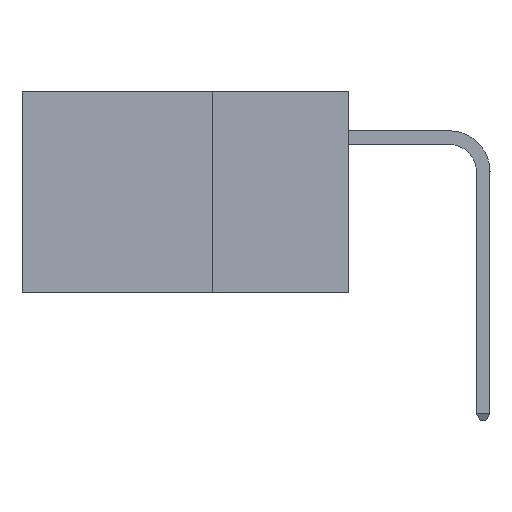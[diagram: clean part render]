
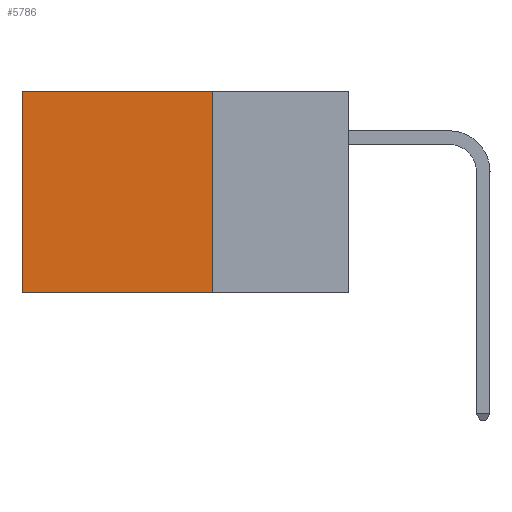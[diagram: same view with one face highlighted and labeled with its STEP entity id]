
A CAD part, left-side view. The second image highlights one B-rep face of the part: STEP entity #5786.
In plain terms, the highlighted planar face has unit normal (-1, 0, 0).
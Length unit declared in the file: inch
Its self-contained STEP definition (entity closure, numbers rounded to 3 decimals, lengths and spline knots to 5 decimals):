
#11 = LINE ( 'NONE', #15499, #3559 ) ;
#218 = CARTESIAN_POINT ( 'NONE',  ( 0.2875, 0.25, -0.37 ) ) ;
#1073 = ORIENTED_EDGE ( 'NONE', *, *, #3732, .F. ) ;
#1570 = CARTESIAN_POINT ( 'NONE',  ( 0.2875, 0.25, -0.37 ) ) ;
#1574 = DIRECTION ( 'NONE',  ( 0., 1., 0. ) ) ;
#2336 = CARTESIAN_POINT ( 'NONE',  ( 0.2875, 0.25, 0. ) ) ;
#2422 = ORIENTED_EDGE ( 'NONE', *, *, #4078, .T. ) ;
#3461 = VERTEX_POINT ( 'NONE', #1570 ) ;
#3559 = VECTOR ( 'NONE', #9134, 39.37008 ) ;
#3732 = EDGE_CURVE ( 'NONE', #3461, #15895, #15954, .T. ) ;
#3923 = AXIS2_PLACEMENT_3D ( 'NONE', #5765, #12413, #4480 ) ;
#4078 = EDGE_CURVE ( 'NONE', #9312, #11743, #8239, .T. ) ;
#4480 = DIRECTION ( 'NONE',  ( 0., 0., -1. ) ) ;
#4950 = CARTESIAN_POINT ( 'NONE',  ( 0.2875, 0.25, 0. ) ) ;
#5463 = CARTESIAN_POINT ( 'NONE',  ( 0.2875, 0.6, 0. ) ) ;
#5624 = EDGE_CURVE ( 'NONE', #11743, #15895, #12311, .T. ) ;
#5765 = CARTESIAN_POINT ( 'NONE',  ( 0.2875, 0.25, 0. ) ) ;
#5786 = ADVANCED_FACE ( 'NONE', ( #12882 ), #9780, .F. ) ;
#6080 = ORIENTED_EDGE ( 'NONE', *, *, #13613, .F. ) ;
#6471 = CARTESIAN_POINT ( 'NONE',  ( 0.2875, 0.6, 0. ) ) ;
#8239 = LINE ( 'NONE', #4950, #11381 ) ;
#9134 = DIRECTION ( 'NONE',  ( 0., 0., -1. ) ) ;
#9312 = VERTEX_POINT ( 'NONE', #2336 ) ;
#9780 = PLANE ( 'NONE',  #3923 ) ;
#11381 = VECTOR ( 'NONE', #14173, 39.37008 ) ;
#11743 = VERTEX_POINT ( 'NONE', #6471 ) ;
#12311 = LINE ( 'NONE', #5463, #15204 ) ;
#12413 = DIRECTION ( 'NONE',  ( 1., 0., 0. ) ) ;
#12640 = EDGE_LOOP ( 'NONE', ( #15151, #1073, #6080, #2422 ) ) ;
#12677 = VECTOR ( 'NONE', #1574, 39.37008 ) ;
#12882 = FACE_OUTER_BOUND ( 'NONE', #12640, .T. ) ;
#13347 = DIRECTION ( 'NONE',  ( 0., 0., -1. ) ) ;
#13613 = EDGE_CURVE ( 'NONE', #9312, #3461, #11, .T. ) ;
#14173 = DIRECTION ( 'NONE',  ( 0., 1., 0. ) ) ;
#15151 = ORIENTED_EDGE ( 'NONE', *, *, #5624, .T. ) ;
#15204 = VECTOR ( 'NONE', #13347, 39.37008 ) ;
#15499 = CARTESIAN_POINT ( 'NONE',  ( 0.2875, 0.25, 0. ) ) ;
#15895 = VERTEX_POINT ( 'NONE', #16261 ) ;
#15954 = LINE ( 'NONE', #218, #12677 ) ;
#16261 = CARTESIAN_POINT ( 'NONE',  ( 0.2875, 0.6, -0.37 ) ) ;
